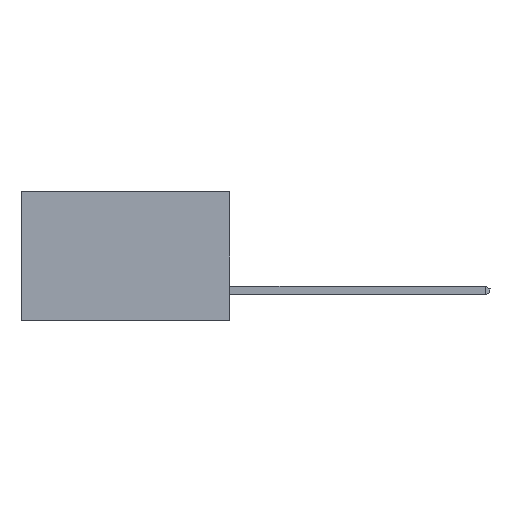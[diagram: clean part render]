
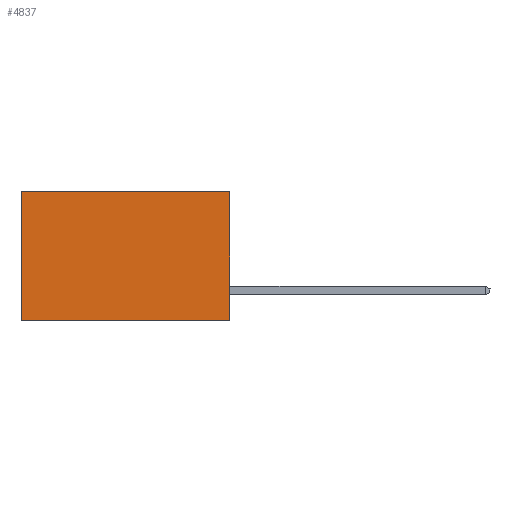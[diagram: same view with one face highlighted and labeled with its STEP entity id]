
A CAD part, left-side view. The second image highlights one B-rep face of the part: STEP entity #4837.
In plain terms, the highlighted planar face has unit normal (-1, 0, 0).
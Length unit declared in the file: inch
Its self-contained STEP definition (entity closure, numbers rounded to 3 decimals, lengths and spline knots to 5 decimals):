
#79 = LINE ( 'NONE', #9385, #1980 ) ;
#711 = LINE ( 'NONE', #3883, #10444 ) ;
#819 = CARTESIAN_POINT ( 'NONE',  ( 0.2615, 0., -0.37 ) ) ;
#1198 = DIRECTION ( 'NONE',  ( 0., 1., 0. ) ) ;
#1251 = DIRECTION ( 'NONE',  ( 0., 0., -1. ) ) ;
#1292 = EDGE_CURVE ( 'NONE', #8167, #4924, #1548, .T. ) ;
#1376 = VERTEX_POINT ( 'NONE', #4015 ) ;
#1548 = LINE ( 'NONE', #5625, #10763 ) ;
#1685 = ORIENTED_EDGE ( 'NONE', *, *, #1292, .F. ) ;
#1795 = CARTESIAN_POINT ( 'NONE',  ( 0.2615, 0., 0. ) ) ;
#1980 = VECTOR ( 'NONE', #1251, 39.37008 ) ;
#2357 = EDGE_LOOP ( 'NONE', ( #11590, #3748, #1685, #6717 ) ) ;
#2762 = CARTESIAN_POINT ( 'NONE',  ( 0.2615, 0.6, 0. ) ) ;
#3600 = DIRECTION ( 'NONE',  ( 1., 0., 0. ) ) ;
#3748 = ORIENTED_EDGE ( 'NONE', *, *, #11589, .F. ) ;
#3750 = DIRECTION ( 'NONE',  ( 0., 0., -1. ) ) ;
#3883 = CARTESIAN_POINT ( 'NONE',  ( 0.2615, 0., -0.37 ) ) ;
#4015 = CARTESIAN_POINT ( 'NONE',  ( 0.2615, 0.6, -0.37 ) ) ;
#4369 = CARTESIAN_POINT ( 'NONE',  ( 0.2615, 0., 0. ) ) ;
#4637 = PLANE ( 'NONE',  #12790 ) ;
#4837 = ADVANCED_FACE ( 'NONE', ( #6706 ), #4637, .F. ) ;
#4924 = VERTEX_POINT ( 'NONE', #819 ) ;
#5625 = CARTESIAN_POINT ( 'NONE',  ( 0.2615, 0., -0.37 ) ) ;
#6270 = EDGE_CURVE ( 'NONE', #10768, #1376, #79, .T. ) ;
#6706 = FACE_OUTER_BOUND ( 'NONE', #2357, .T. ) ;
#6717 = ORIENTED_EDGE ( 'NONE', *, *, #7952, .T. ) ;
#6773 = DIRECTION ( 'NONE',  ( 0., 0., -1. ) ) ;
#7778 = DIRECTION ( 'NONE',  ( 0., 1., 0. ) ) ;
#7952 = EDGE_CURVE ( 'NONE', #8167, #10768, #13452, .T. ) ;
#8167 = VERTEX_POINT ( 'NONE', #1795 ) ;
#8851 = CARTESIAN_POINT ( 'NONE',  ( 0.2615, 0., -0.37 ) ) ;
#9385 = CARTESIAN_POINT ( 'NONE',  ( 0.2615, 0.6, -0.37 ) ) ;
#9528 = VECTOR ( 'NONE', #1198, 39.37008 ) ;
#10444 = VECTOR ( 'NONE', #7778, 39.37008 ) ;
#10763 = VECTOR ( 'NONE', #3750, 39.37008 ) ;
#10768 = VERTEX_POINT ( 'NONE', #2762 ) ;
#11589 = EDGE_CURVE ( 'NONE', #4924, #1376, #711, .T. ) ;
#11590 = ORIENTED_EDGE ( 'NONE', *, *, #6270, .T. ) ;
#12790 = AXIS2_PLACEMENT_3D ( 'NONE', #8851, #3600, #6773 ) ;
#13452 = LINE ( 'NONE', #4369, #9528 ) ;
